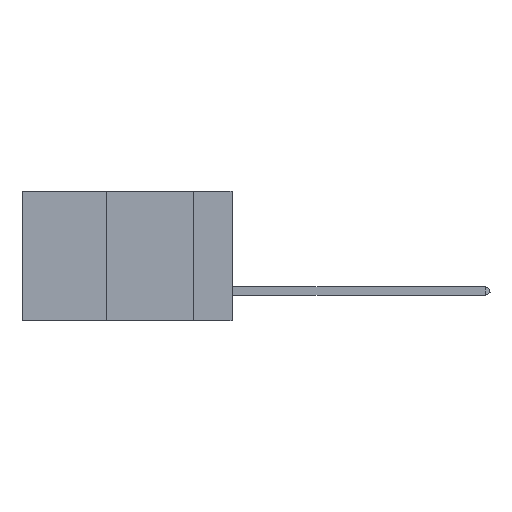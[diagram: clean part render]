
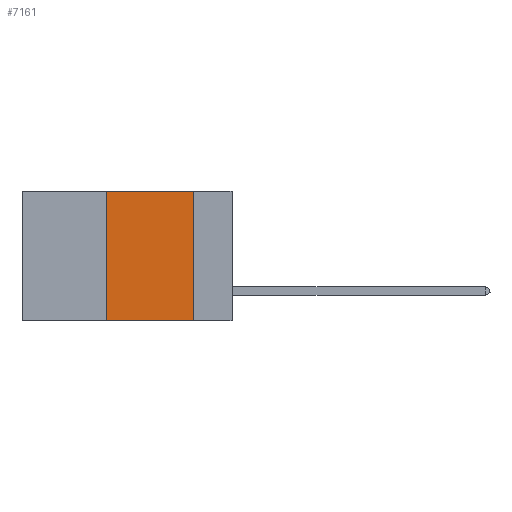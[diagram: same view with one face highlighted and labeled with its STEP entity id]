
A CAD part, left-side view. The second image highlights one B-rep face of the part: STEP entity #7161.
In plain terms, the highlighted planar face has unit normal (-1, 0, 0).
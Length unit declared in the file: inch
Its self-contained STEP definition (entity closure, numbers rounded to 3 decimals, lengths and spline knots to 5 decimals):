
#745 = DIRECTION ( 'NONE',  ( 0., -1., 0. ) ) ;
#2847 = CARTESIAN_POINT ( 'NONE',  ( 0., 0.11, 0. ) ) ;
#3485 = VECTOR ( 'NONE', #24162, 39.37008 ) ;
#3611 = LINE ( 'NONE', #9925, #21250 ) ;
#3745 = CARTESIAN_POINT ( 'NONE',  ( 0., 0.36, 0. ) ) ;
#5463 = ORIENTED_EDGE ( 'NONE', *, *, #11311, .F. ) ;
#5979 = LINE ( 'NONE', #10167, #3485 ) ;
#7161 = ADVANCED_FACE ( 'NONE', ( #17048 ), #28635, .F. ) ;
#8996 = DIRECTION ( 'NONE',  ( 0., -1., 0. ) ) ;
#9925 = CARTESIAN_POINT ( 'NONE',  ( 0., 0.6, -0.37 ) ) ;
#9998 = VERTEX_POINT ( 'NONE', #2847 ) ;
#10167 = CARTESIAN_POINT ( 'NONE',  ( 0., 0.11, 0. ) ) ;
#10862 = EDGE_CURVE ( 'NONE', #9998, #26606, #5979, .T. ) ;
#11311 = EDGE_CURVE ( 'NONE', #11521, #26043, #12578, .T. ) ;
#11521 = VERTEX_POINT ( 'NONE', #19041 ) ;
#11891 = EDGE_CURVE ( 'NONE', #26043, #9998, #17595, .T. ) ;
#12578 = LINE ( 'NONE', #3745, #17286 ) ;
#14209 = ORIENTED_EDGE ( 'NONE', *, *, #10862, .F. ) ;
#17048 = FACE_OUTER_BOUND ( 'NONE', #19377, .T. ) ;
#17072 = EDGE_CURVE ( 'NONE', #11521, #26606, #3611, .T. ) ;
#17250 = AXIS2_PLACEMENT_3D ( 'NONE', #28731, #19622, #19711 ) ;
#17286 = VECTOR ( 'NONE', #24606, 39.37008 ) ;
#17595 = LINE ( 'NONE', #22357, #19732 ) ;
#19041 = CARTESIAN_POINT ( 'NONE',  ( 0., 0.36, -0.37 ) ) ;
#19377 = EDGE_LOOP ( 'NONE', ( #14209, #26498, #5463, #25199 ) ) ;
#19622 = DIRECTION ( 'NONE',  ( 1., 0., 0. ) ) ;
#19711 = DIRECTION ( 'NONE',  ( 0., 0., -1. ) ) ;
#19732 = VECTOR ( 'NONE', #8996, 39.37008 ) ;
#21250 = VECTOR ( 'NONE', #745, 39.37008 ) ;
#22357 = CARTESIAN_POINT ( 'NONE',  ( 0., 0.6, 0. ) ) ;
#24162 = DIRECTION ( 'NONE',  ( 0., 0., -1. ) ) ;
#24289 = CARTESIAN_POINT ( 'NONE',  ( 0., 0.11, -0.37 ) ) ;
#24606 = DIRECTION ( 'NONE',  ( 0., 0., 1. ) ) ;
#25199 = ORIENTED_EDGE ( 'NONE', *, *, #17072, .T. ) ;
#26043 = VERTEX_POINT ( 'NONE', #29133 ) ;
#26498 = ORIENTED_EDGE ( 'NONE', *, *, #11891, .F. ) ;
#26606 = VERTEX_POINT ( 'NONE', #24289 ) ;
#28635 = PLANE ( 'NONE',  #17250 ) ;
#28731 = CARTESIAN_POINT ( 'NONE',  ( 0., 0.6, 0. ) ) ;
#29133 = CARTESIAN_POINT ( 'NONE',  ( 0., 0.36, 0. ) ) ;
